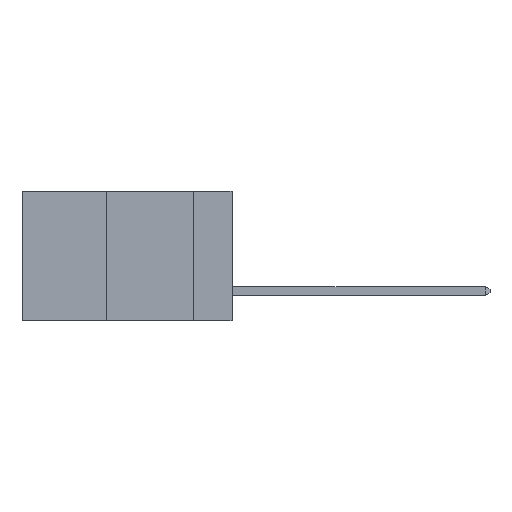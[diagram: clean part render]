
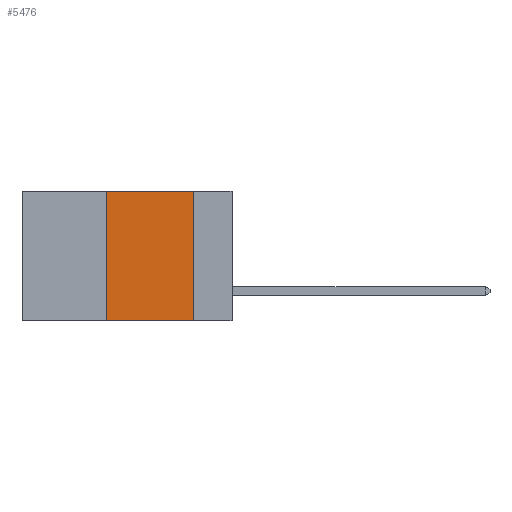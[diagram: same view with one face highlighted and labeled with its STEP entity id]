
A CAD part, left-side view. The second image highlights one B-rep face of the part: STEP entity #5476.
In plain terms, the highlighted planar face has unit normal (-1, 0, 0).
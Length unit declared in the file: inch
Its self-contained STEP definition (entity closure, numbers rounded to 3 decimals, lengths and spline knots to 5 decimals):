
#29 = EDGE_CURVE ( 'NONE', #9551, #7683, #2987, .T. ) ;
#1673 = VECTOR ( 'NONE', #12968, 39.37008 ) ;
#1902 = CARTESIAN_POINT ( 'NONE',  ( 0., 0.6, 0. ) ) ;
#2826 = ORIENTED_EDGE ( 'NONE', *, *, #29, .T. ) ;
#2897 = VERTEX_POINT ( 'NONE', #5171 ) ;
#2987 = LINE ( 'NONE', #15408, #15722 ) ;
#3007 = LINE ( 'NONE', #6031, #13299 ) ;
#3313 = ORIENTED_EDGE ( 'NONE', *, *, #13345, .F. ) ;
#5171 = CARTESIAN_POINT ( 'NONE',  ( 0., 0.36, 0. ) ) ;
#5476 = ADVANCED_FACE ( 'NONE', ( #11443 ), #12346, .F. ) ;
#6031 = CARTESIAN_POINT ( 'NONE',  ( 0., 0.11, 0. ) ) ;
#6593 = VECTOR ( 'NONE', #10703, 39.37008 ) ;
#6867 = CARTESIAN_POINT ( 'NONE',  ( 0., 0.11, -0.37 ) ) ;
#7421 = DIRECTION ( 'NONE',  ( 1., 0., 0. ) ) ;
#7683 = VERTEX_POINT ( 'NONE', #6867 ) ;
#7967 = AXIS2_PLACEMENT_3D ( 'NONE', #12293, #7421, #15962 ) ;
#9551 = VERTEX_POINT ( 'NONE', #12423 ) ;
#9637 = EDGE_LOOP ( 'NONE', ( #10800, #3313, #10992, #2826 ) ) ;
#10703 = DIRECTION ( 'NONE',  ( 0., -1., 0. ) ) ;
#10800 = ORIENTED_EDGE ( 'NONE', *, *, #14416, .F. ) ;
#10992 = ORIENTED_EDGE ( 'NONE', *, *, #12690, .F. ) ;
#11443 = FACE_OUTER_BOUND ( 'NONE', #9637, .T. ) ;
#11683 = LINE ( 'NONE', #11770, #1673 ) ;
#11770 = CARTESIAN_POINT ( 'NONE',  ( 0., 0.36, 0. ) ) ;
#12293 = CARTESIAN_POINT ( 'NONE',  ( 0., 0.6, 0. ) ) ;
#12346 = PLANE ( 'NONE',  #7967 ) ;
#12423 = CARTESIAN_POINT ( 'NONE',  ( 0., 0.36, -0.37 ) ) ;
#12690 = EDGE_CURVE ( 'NONE', #9551, #2897, #11683, .T. ) ;
#12968 = DIRECTION ( 'NONE',  ( 0., 0., 1. ) ) ;
#13299 = VECTOR ( 'NONE', #14596, 39.37008 ) ;
#13345 = EDGE_CURVE ( 'NONE', #2897, #14800, #15965, .T. ) ;
#14074 = CARTESIAN_POINT ( 'NONE',  ( 0., 0.11, 0. ) ) ;
#14416 = EDGE_CURVE ( 'NONE', #14800, #7683, #3007, .T. ) ;
#14596 = DIRECTION ( 'NONE',  ( 0., 0., -1. ) ) ;
#14800 = VERTEX_POINT ( 'NONE', #14074 ) ;
#15277 = DIRECTION ( 'NONE',  ( 0., -1., 0. ) ) ;
#15408 = CARTESIAN_POINT ( 'NONE',  ( 0., 0.6, -0.37 ) ) ;
#15722 = VECTOR ( 'NONE', #15277, 39.37008 ) ;
#15962 = DIRECTION ( 'NONE',  ( 0., 0., -1. ) ) ;
#15965 = LINE ( 'NONE', #1902, #6593 ) ;
